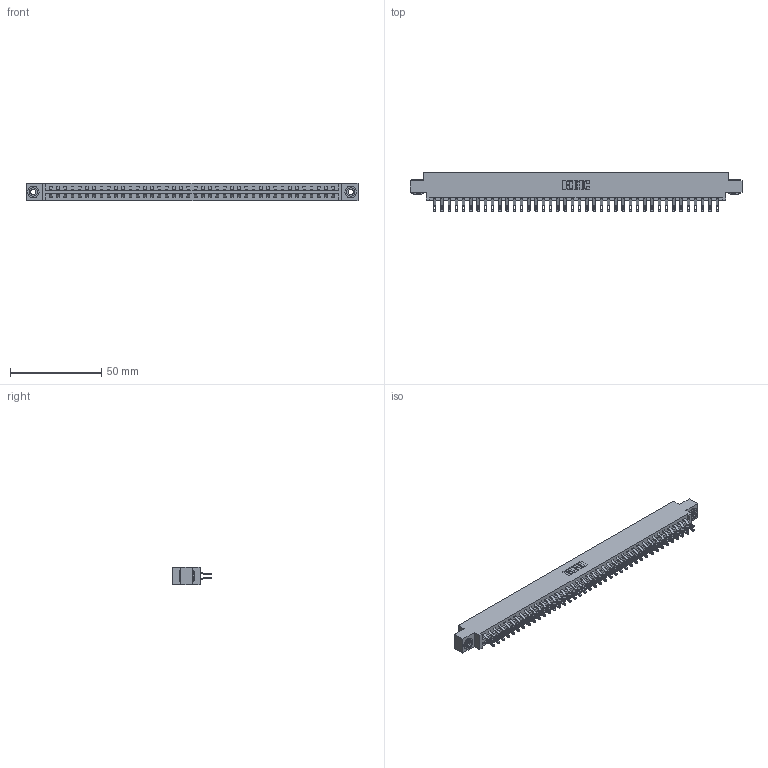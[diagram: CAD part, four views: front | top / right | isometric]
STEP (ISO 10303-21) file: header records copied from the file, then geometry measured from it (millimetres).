
FILE_DESCRIPTION (( 'STEP AP203' ), '1' );
FILE_NAME ('337-080-555-803.STEP', '2019-10-15T15:32:53', ( '' ), ( '' ), 'SwSTEP 2.0', 'SolidWorks 2016', '' );
FILE_SCHEMA (( 'CONFIG_CONTROL_DESIGN' ));
Length unit declared in the file: inch
Products named in the file (4): 337 Part_0.170 Offset - 0.156 Dia-TH; 345-250-002_345-250-002-102; 345-292-001_555 Tail; 337-080-555-803
Assembly tree (83 placements, depth 2):
  337-080-555-803
    337 Part_0.170 Offset - 0.156 Dia-TH
    345-292-001_555 Tail  x80
    345-250-002_345-250-002-102  x2
Bounding box: 181.51 x 21.47 x 9.4 mm (x, y, z)
Volume: 19236.1 mm3; surface area: 22933.7 mm2
Topology: 83 solids, 83 shells, 4956 faces, 15519 edges, 10342 vertices
Faces by surface type: plane 2964, cylinder 1984, cone 8
Entity records: 32380 total; most frequent: CARTESIAN_POINT 5467, ORIENTED_EDGE 5366, DIRECTION 4657, EDGE_CURVE 2683, VECTOR 2511, LINE 2511, VERTEX_POINT 1786, AXIS2_PLACEMENT_3D 1073
